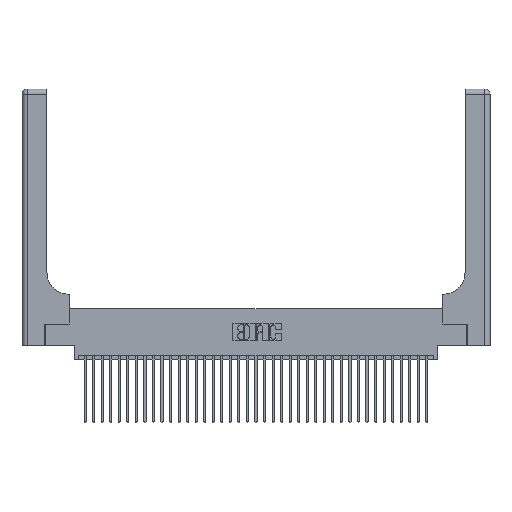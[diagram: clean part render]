
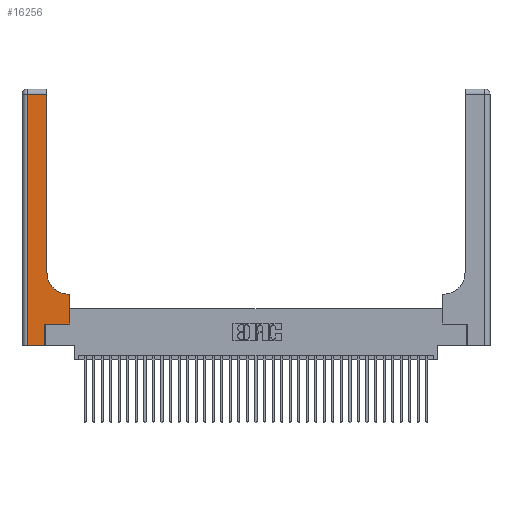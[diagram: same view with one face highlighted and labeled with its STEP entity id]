
A CAD part, top view. The second image highlights one B-rep face of the part: STEP entity #16256.
In plain terms, the highlighted planar face has unit normal (0, 0, 1).
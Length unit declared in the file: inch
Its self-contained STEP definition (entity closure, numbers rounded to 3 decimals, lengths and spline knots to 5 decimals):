
#91 = AXIS2_PLACEMENT_3D ( 'NONE', #17530, #23627, #26422 ) ;
#246 = LINE ( 'NONE', #25671, #2970 ) ;
#307 = ORIENTED_EDGE ( 'NONE', *, *, #14620, .T. ) ;
#994 = VERTEX_POINT ( 'NONE', #5473 ) ;
#1073 = LINE ( 'NONE', #10830, #17002 ) ;
#1164 = EDGE_LOOP ( 'NONE', ( #24535, #307, #24455, #24720, #33660, #16169, #25443, #15723, #3953 ) ) ;
#1810 = VECTOR ( 'NONE', #36657, 39.37008 ) ;
#1817 = CARTESIAN_POINT ( 'NONE',  ( 0.269, 0., 0.37 ) ) ;
#1907 = DIRECTION ( 'NONE',  ( 0., 1., 0. ) ) ;
#2391 = VERTEX_POINT ( 'NONE', #22560 ) ;
#2485 = DIRECTION ( 'NONE',  ( -1., 0., 0. ) ) ;
#2970 = VECTOR ( 'NONE', #2485, 39.37008 ) ;
#3259 = VERTEX_POINT ( 'NONE', #26276 ) ;
#3292 = CARTESIAN_POINT ( 'NONE',  ( 0., 0., 0.37 ) ) ;
#3419 = LINE ( 'NONE', #17161, #23464 ) ;
#3953 = ORIENTED_EDGE ( 'NONE', *, *, #5511, .T. ) ;
#4735 = CARTESIAN_POINT ( 'NONE',  ( 0.5415, 0.85, 0.37 ) ) ;
#4852 = VERTEX_POINT ( 'NONE', #21808 ) ;
#5081 = CARTESIAN_POINT ( 'NONE',  ( 0.2915, 3., 0.37 ) ) ;
#5284 = DIRECTION ( 'NONE',  ( 1., 0., 0. ) ) ;
#5473 = CARTESIAN_POINT ( 'NONE',  ( 0.269, 0.25, 0.37 ) ) ;
#5511 = EDGE_CURVE ( 'NONE', #25549, #16251, #36893, .T. ) ;
#5657 = CARTESIAN_POINT ( 'NONE',  ( 0.2915, 0.85, 0.37 ) ) ;
#6037 = LINE ( 'NONE', #18389, #30665 ) ;
#6486 = EDGE_CURVE ( 'NONE', #3259, #31445, #12329, .T. ) ;
#6721 = VECTOR ( 'NONE', #1907, 39.37008 ) ;
#9011 = CARTESIAN_POINT ( 'NONE',  ( 0.269, 0., 0.37 ) ) ;
#9707 = CARTESIAN_POINT ( 'NONE',  ( 0.5585, 0.25, 0.37 ) ) ;
#10210 = DIRECTION ( 'NONE',  ( 1., 0., 0. ) ) ;
#10349 = VERTEX_POINT ( 'NONE', #1817 ) ;
#10830 = CARTESIAN_POINT ( 'NONE',  ( 0.5585, 0.25, 0.37 ) ) ;
#12329 = LINE ( 'NONE', #16127, #1810 ) ;
#12375 = FACE_OUTER_BOUND ( 'NONE', #1164, .T. ) ;
#14620 = EDGE_CURVE ( 'NONE', #2391, #3259, #6037, .T. ) ;
#15723 = ORIENTED_EDGE ( 'NONE', *, *, #27766, .T. ) ;
#16127 = CARTESIAN_POINT ( 'NONE',  ( 0.06, 3., 0.37 ) ) ;
#16169 = ORIENTED_EDGE ( 'NONE', *, *, #27740, .T. ) ;
#16251 = VERTEX_POINT ( 'NONE', #5657 ) ;
#16256 = ADVANCED_FACE ( 'NONE', ( #12375 ), #19836, .F. ) ;
#17002 = VECTOR ( 'NONE', #25862, 39.37008 ) ;
#17161 = CARTESIAN_POINT ( 'NONE',  ( 0.269, 0.25, 0.37 ) ) ;
#17530 = CARTESIAN_POINT ( 'NONE',  ( 0., 3., 0.37 ) ) ;
#18389 = CARTESIAN_POINT ( 'NONE',  ( 0., 2.94, 0.37 ) ) ;
#19287 = DIRECTION ( 'NONE',  ( 0., 0., -1. ) ) ;
#19836 = PLANE ( 'NONE',  #91 ) ;
#21297 = LINE ( 'NONE', #9011, #34879 ) ;
#21447 = VECTOR ( 'NONE', #29130, 39.37008 ) ;
#21585 = EDGE_CURVE ( 'NONE', #10349, #994, #21297, .T. ) ;
#21808 = CARTESIAN_POINT ( 'NONE',  ( 0.5585, 0.6, 0.37 ) ) ;
#22560 = CARTESIAN_POINT ( 'NONE',  ( 0.2915, 2.94, 0.37 ) ) ;
#23464 = VECTOR ( 'NONE', #5284, 39.37008 ) ;
#23627 = DIRECTION ( 'NONE',  ( 0., 0., -1. ) ) ;
#24455 = ORIENTED_EDGE ( 'NONE', *, *, #6486, .T. ) ;
#24535 = ORIENTED_EDGE ( 'NONE', *, *, #26845, .T. ) ;
#24720 = ORIENTED_EDGE ( 'NONE', *, *, #34720, .T. ) ;
#25443 = ORIENTED_EDGE ( 'NONE', *, *, #30174, .T. ) ;
#25549 = VERTEX_POINT ( 'NONE', #35991 ) ;
#25671 = CARTESIAN_POINT ( 'NONE',  ( 0.2915, 0.6, 0.37 ) ) ;
#25862 = DIRECTION ( 'NONE',  ( 0., 1., 0. ) ) ;
#26168 = VERTEX_POINT ( 'NONE', #9707 ) ;
#26276 = CARTESIAN_POINT ( 'NONE',  ( 0.06, 2.94, 0.37 ) ) ;
#26282 = LINE ( 'NONE', #5081, #6721 ) ;
#26422 = DIRECTION ( 'NONE',  ( -1., 0., 0. ) ) ;
#26711 = AXIS2_PLACEMENT_3D ( 'NONE', #4735, #19287, #10210 ) ;
#26845 = EDGE_CURVE ( 'NONE', #16251, #2391, #26282, .T. ) ;
#27740 = EDGE_CURVE ( 'NONE', #994, #26168, #3419, .T. ) ;
#27766 = EDGE_CURVE ( 'NONE', #4852, #25549, #246, .T. ) ;
#29130 = DIRECTION ( 'NONE',  ( 1., 0., 0. ) ) ;
#30174 = EDGE_CURVE ( 'NONE', #26168, #4852, #1073, .T. ) ;
#30665 = VECTOR ( 'NONE', #32750, 39.37008 ) ;
#31445 = VERTEX_POINT ( 'NONE', #37028 ) ;
#32750 = DIRECTION ( 'NONE',  ( -1., 0., 0. ) ) ;
#33660 = ORIENTED_EDGE ( 'NONE', *, *, #21585, .T. ) ;
#34720 = EDGE_CURVE ( 'NONE', #31445, #10349, #35048, .T. ) ;
#34879 = VECTOR ( 'NONE', #35090, 39.37008 ) ;
#35048 = LINE ( 'NONE', #3292, #21447 ) ;
#35090 = DIRECTION ( 'NONE',  ( 0., 1., 0. ) ) ;
#35991 = CARTESIAN_POINT ( 'NONE',  ( 0.5415, 0.6, 0.37 ) ) ;
#36657 = DIRECTION ( 'NONE',  ( 0., -1., 0. ) ) ;
#36893 = CIRCLE ( 'NONE', #26711, 0.25 ) ;
#37028 = CARTESIAN_POINT ( 'NONE',  ( 0.06, 0., 0.37 ) ) ;
